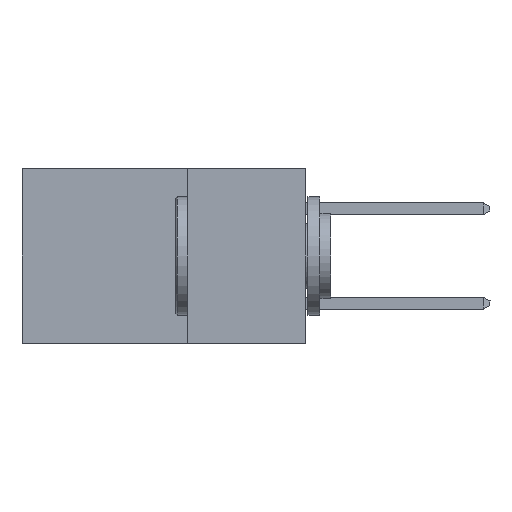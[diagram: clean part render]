
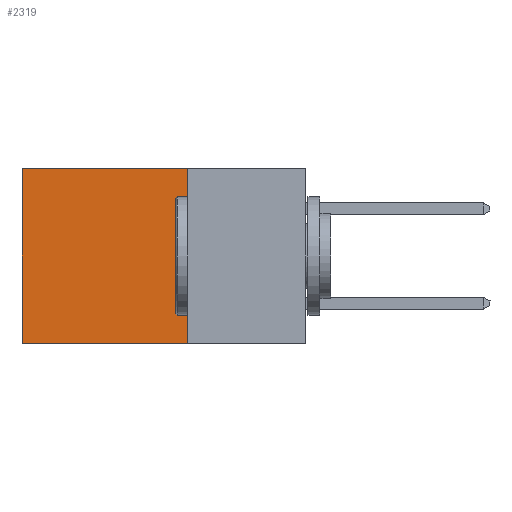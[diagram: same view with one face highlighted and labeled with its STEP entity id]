
A CAD part, left-side view. The second image highlights one B-rep face of the part: STEP entity #2319.
In plain terms, the highlighted planar face has unit normal (-1, 0, 0).
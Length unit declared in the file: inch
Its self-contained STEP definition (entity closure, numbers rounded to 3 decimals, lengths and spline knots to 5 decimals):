
#147 = EDGE_CURVE ( 'NONE', #1315, #11095, #2904, .T. ) ;
#404 = DIRECTION ( 'NONE',  ( 0., 0., -1. ) ) ;
#533 = DIRECTION ( 'NONE',  ( 0., 0., -1. ) ) ;
#735 = CARTESIAN_POINT ( 'NONE',  ( 0.298, 0.25, 0. ) ) ;
#791 = DIRECTION ( 'NONE',  ( 0., 1., 0. ) ) ;
#1315 = VERTEX_POINT ( 'NONE', #8112 ) ;
#1996 = FACE_OUTER_BOUND ( 'NONE', #7290, .T. ) ;
#2174 = DIRECTION ( 'NONE',  ( 0., 0., -1. ) ) ;
#2319 = ADVANCED_FACE ( 'NONE', ( #1996 ), #2457, .F. ) ;
#2457 = PLANE ( 'NONE',  #5348 ) ;
#2502 = CARTESIAN_POINT ( 'NONE',  ( 0.298, 0.25, 0. ) ) ;
#2743 = ORIENTED_EDGE ( 'NONE', *, *, #147, .F. ) ;
#2904 = LINE ( 'NONE', #5586, #10244 ) ;
#3870 = CARTESIAN_POINT ( 'NONE',  ( 0.298, 0.6, 0. ) ) ;
#4156 = CARTESIAN_POINT ( 'NONE',  ( 0.298, 0.25, 0. ) ) ;
#4325 = ORIENTED_EDGE ( 'NONE', *, *, #7199, .T. ) ;
#4727 = ORIENTED_EDGE ( 'NONE', *, *, #6949, .F. ) ;
#5291 = CARTESIAN_POINT ( 'NONE',  ( 0.298, 0.25, 0. ) ) ;
#5348 = AXIS2_PLACEMENT_3D ( 'NONE', #4156, #6007, #404 ) ;
#5586 = CARTESIAN_POINT ( 'NONE',  ( 0.298, 0.25, -0.37 ) ) ;
#6007 = DIRECTION ( 'NONE',  ( 1., 0., 0. ) ) ;
#6501 = DIRECTION ( 'NONE',  ( 0., 1., 0. ) ) ;
#6559 = LINE ( 'NONE', #2502, #11147 ) ;
#6686 = LINE ( 'NONE', #9429, #8977 ) ;
#6949 = EDGE_CURVE ( 'NONE', #10773, #1315, #6559, .T. ) ;
#6993 = LINE ( 'NONE', #735, #7275 ) ;
#7199 = EDGE_CURVE ( 'NONE', #10773, #11584, #6993, .T. ) ;
#7275 = VECTOR ( 'NONE', #791, 39.37008 ) ;
#7290 = EDGE_LOOP ( 'NONE', ( #8750, #2743, #4727, #4325 ) ) ;
#8112 = CARTESIAN_POINT ( 'NONE',  ( 0.298, 0.25, -0.37 ) ) ;
#8750 = ORIENTED_EDGE ( 'NONE', *, *, #11667, .T. ) ;
#8977 = VECTOR ( 'NONE', #2174, 39.37008 ) ;
#9429 = CARTESIAN_POINT ( 'NONE',  ( 0.298, 0.6, 0. ) ) ;
#10244 = VECTOR ( 'NONE', #6501, 39.37008 ) ;
#10315 = CARTESIAN_POINT ( 'NONE',  ( 0.298, 0.6, -0.37 ) ) ;
#10773 = VERTEX_POINT ( 'NONE', #5291 ) ;
#11095 = VERTEX_POINT ( 'NONE', #10315 ) ;
#11147 = VECTOR ( 'NONE', #533, 39.37008 ) ;
#11584 = VERTEX_POINT ( 'NONE', #3870 ) ;
#11667 = EDGE_CURVE ( 'NONE', #11584, #11095, #6686, .T. ) ;
